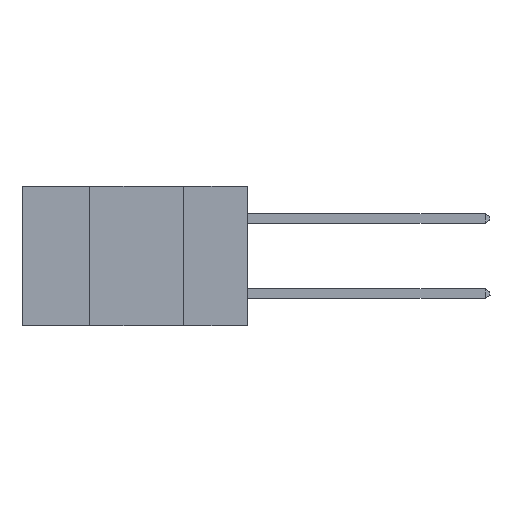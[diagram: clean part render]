
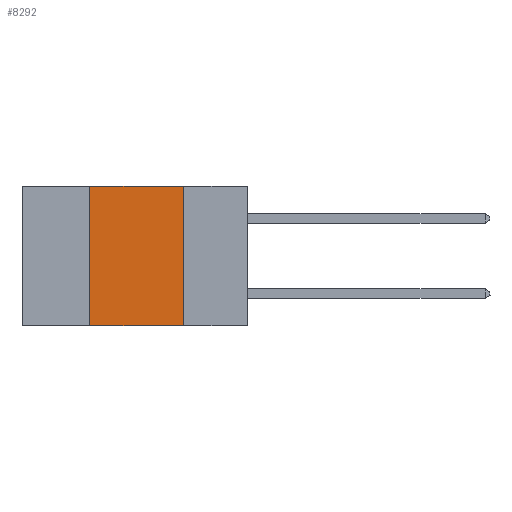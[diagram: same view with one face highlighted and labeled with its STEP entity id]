
A CAD part, left-side view. The second image highlights one B-rep face of the part: STEP entity #8292.
In plain terms, the highlighted planar face has unit normal (-1, 0, 0).
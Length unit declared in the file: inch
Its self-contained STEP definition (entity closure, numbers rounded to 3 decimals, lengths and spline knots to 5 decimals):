
#631 = EDGE_CURVE ( 'NONE', #6214, #6795, #15228, .T. ) ;
#776 = ORIENTED_EDGE ( 'NONE', *, *, #5217, .F. ) ;
#997 = CARTESIAN_POINT ( 'NONE',  ( 0., 0.6, 0. ) ) ;
#1130 = CARTESIAN_POINT ( 'NONE',  ( 0., 0.6, -0.37 ) ) ;
#1724 = CARTESIAN_POINT ( 'NONE',  ( 0., 0.17, 0. ) ) ;
#1843 = LINE ( 'NONE', #1130, #11019 ) ;
#2529 = EDGE_CURVE ( 'NONE', #6214, #5466, #1843, .T. ) ;
#2726 = PLANE ( 'NONE',  #10127 ) ;
#3053 = CARTESIAN_POINT ( 'NONE',  ( 0., 0.42, 0. ) ) ;
#3385 = VECTOR ( 'NONE', #13766, 39.37008 ) ;
#3775 = DIRECTION ( 'NONE',  ( 0., -1., 0. ) ) ;
#4160 = DIRECTION ( 'NONE',  ( 0., 0., -1. ) ) ;
#5022 = CARTESIAN_POINT ( 'NONE',  ( 0., 0.42, 0. ) ) ;
#5217 = EDGE_CURVE ( 'NONE', #13188, #5466, #11742, .T. ) ;
#5466 = VERTEX_POINT ( 'NONE', #16808 ) ;
#6214 = VERTEX_POINT ( 'NONE', #13786 ) ;
#6795 = VERTEX_POINT ( 'NONE', #5022 ) ;
#7190 = LINE ( 'NONE', #997, #16122 ) ;
#7619 = DIRECTION ( 'NONE',  ( 0., -1., 0. ) ) ;
#8292 = ADVANCED_FACE ( 'NONE', ( #10817 ), #2726, .F. ) ;
#10127 = AXIS2_PLACEMENT_3D ( 'NONE', #14652, #10792, #4160 ) ;
#10398 = ORIENTED_EDGE ( 'NONE', *, *, #14332, .F. ) ;
#10792 = DIRECTION ( 'NONE',  ( 1., 0., 0. ) ) ;
#10817 = FACE_OUTER_BOUND ( 'NONE', #14201, .T. ) ;
#10848 = ORIENTED_EDGE ( 'NONE', *, *, #2529, .T. ) ;
#11019 = VECTOR ( 'NONE', #3775, 39.37008 ) ;
#11062 = DIRECTION ( 'NONE',  ( 0., 0., -1. ) ) ;
#11742 = LINE ( 'NONE', #1724, #15291 ) ;
#12340 = ORIENTED_EDGE ( 'NONE', *, *, #631, .F. ) ;
#13188 = VERTEX_POINT ( 'NONE', #16233 ) ;
#13766 = DIRECTION ( 'NONE',  ( 0., 0., 1. ) ) ;
#13786 = CARTESIAN_POINT ( 'NONE',  ( 0., 0.42, -0.37 ) ) ;
#14201 = EDGE_LOOP ( 'NONE', ( #776, #10398, #12340, #10848 ) ) ;
#14332 = EDGE_CURVE ( 'NONE', #6795, #13188, #7190, .T. ) ;
#14652 = CARTESIAN_POINT ( 'NONE',  ( 0., 0.6, 0. ) ) ;
#15228 = LINE ( 'NONE', #3053, #3385 ) ;
#15291 = VECTOR ( 'NONE', #11062, 39.37008 ) ;
#16122 = VECTOR ( 'NONE', #7619, 39.37008 ) ;
#16233 = CARTESIAN_POINT ( 'NONE',  ( 0., 0.17, 0. ) ) ;
#16808 = CARTESIAN_POINT ( 'NONE',  ( 0., 0.17, -0.37 ) ) ;
